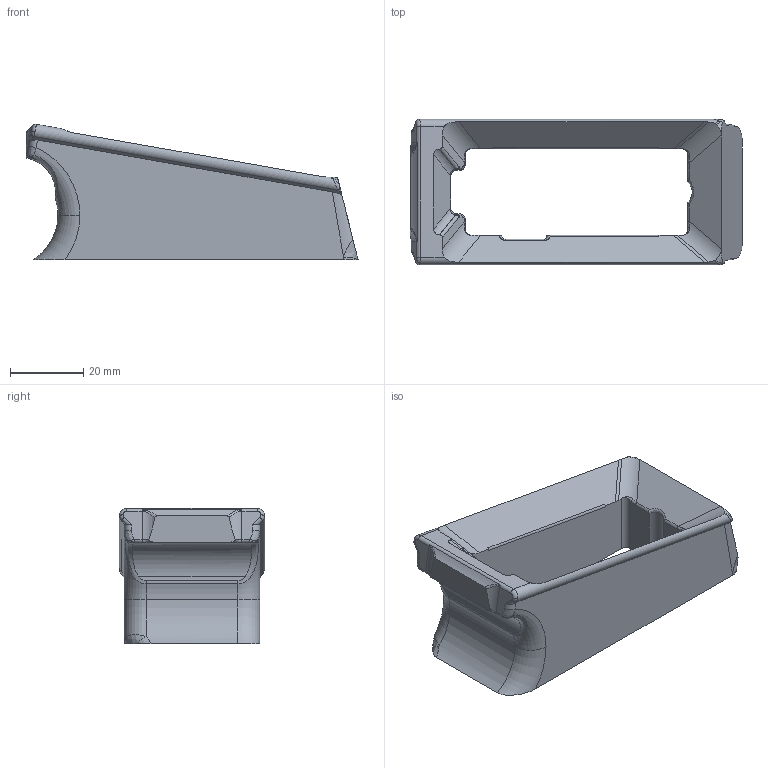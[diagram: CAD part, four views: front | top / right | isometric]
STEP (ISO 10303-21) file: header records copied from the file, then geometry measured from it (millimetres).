
FILE_DESCRIPTION (( 'STEP AP214' ), '1' );
FILE_NAME ('Magwell_3a_1.step', '2019-12-18T03:08:18', ( '' ), ( '' ), 'SwSTEP 2.0', 'SolidWorks 2019', '' );
FILE_SCHEMA (( 'AUTOMOTIVE_DESIGN' ));
Length unit declared in the file: millimetre
Products named in the file (1): Magwell_3a_1
Bounding box: 90.85 x 39.78 x 37.04 mm (x, y, z)
Volume: 39306.8 mm3; surface area: 15067.4 mm2
Topology: 1 solids, 1 shells, 170 faces, 450 edges, 276 vertices
Faces by surface type: bspline 58, cylinder 50, plane 47, torus 13, sphere 2
Entity records: 7854 total; most frequent: CARTESIAN_POINT 4200, ORIENTED_EDGE 890, DIRECTION 598, EDGE_CURVE 445, VERTEX_POINT 276, AXIS2_PLACEMENT_3D 217, EDGE_LOOP 171, FACE_OUTER_BOUND 170
